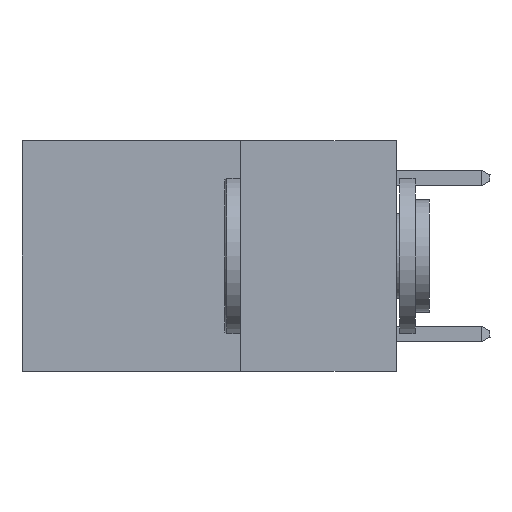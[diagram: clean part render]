
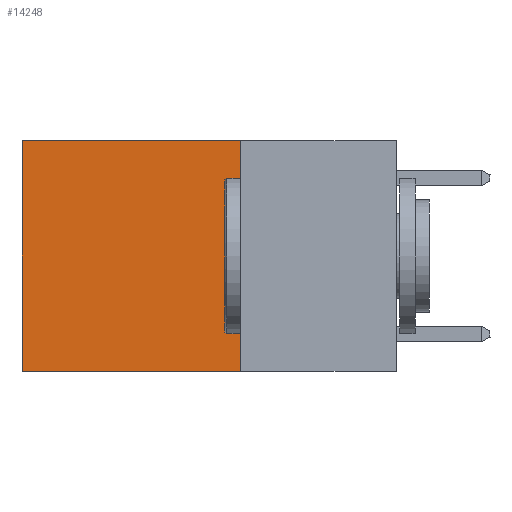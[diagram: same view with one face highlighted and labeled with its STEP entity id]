
A CAD part, left-side view. The second image highlights one B-rep face of the part: STEP entity #14248.
In plain terms, the highlighted planar face has unit normal (-1, 0, 0).
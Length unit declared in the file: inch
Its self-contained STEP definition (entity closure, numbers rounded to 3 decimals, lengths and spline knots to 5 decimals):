
#1672 = EDGE_CURVE ( 'NONE', #14517, #18573, #16495, .T. ) ;
#2757 = LINE ( 'NONE', #18654, #20896 ) ;
#2810 = LINE ( 'NONE', #10852, #20911 ) ;
#2947 = CARTESIAN_POINT ( 'NONE',  ( 0.2625, 0.25, -0.37 ) ) ;
#3266 = DIRECTION ( 'NONE',  ( 0., 0., -1. ) ) ;
#4564 = VERTEX_POINT ( 'NONE', #9710 ) ;
#4929 = DIRECTION ( 'NONE',  ( 0., 1., 0. ) ) ;
#6779 = LINE ( 'NONE', #2947, #18053 ) ;
#7297 = ORIENTED_EDGE ( 'NONE', *, *, #20606, .T. ) ;
#8660 = VERTEX_POINT ( 'NONE', #10521 ) ;
#8842 = DIRECTION ( 'NONE',  ( 0., 0., -1. ) ) ;
#9063 = DIRECTION ( 'NONE',  ( 1., 0., 0. ) ) ;
#9200 = CARTESIAN_POINT ( 'NONE',  ( 0.2625, 0.25, 0. ) ) ;
#9710 = CARTESIAN_POINT ( 'NONE',  ( 0.2625, 0.6, -0.37 ) ) ;
#10521 = CARTESIAN_POINT ( 'NONE',  ( 0.2625, 0.25, -0.37 ) ) ;
#10604 = CARTESIAN_POINT ( 'NONE',  ( 0.2625, 0.25, 0. ) ) ;
#10770 = ORIENTED_EDGE ( 'NONE', *, *, #19066, .F. ) ;
#10775 = EDGE_LOOP ( 'NONE', ( #7297, #10770, #15375, #19429 ) ) ;
#10852 = CARTESIAN_POINT ( 'NONE',  ( 0.2625, 0.6, 0. ) ) ;
#10912 = EDGE_CURVE ( 'NONE', #14517, #8660, #2757, .T. ) ;
#14248 = ADVANCED_FACE ( 'NONE', ( #19027 ), #23471, .F. ) ;
#14517 = VERTEX_POINT ( 'NONE', #10604 ) ;
#14653 = CARTESIAN_POINT ( 'NONE',  ( 0.2625, 0.25, 0. ) ) ;
#15375 = ORIENTED_EDGE ( 'NONE', *, *, #10912, .F. ) ;
#16280 = CARTESIAN_POINT ( 'NONE',  ( 0.2625, 0.6, 0. ) ) ;
#16495 = LINE ( 'NONE', #14653, #22842 ) ;
#18053 = VECTOR ( 'NONE', #20395, 39.37008 ) ;
#18573 = VERTEX_POINT ( 'NONE', #16280 ) ;
#18654 = CARTESIAN_POINT ( 'NONE',  ( 0.2625, 0.25, 0. ) ) ;
#18839 = DIRECTION ( 'NONE',  ( 0., 0., -1. ) ) ;
#19027 = FACE_OUTER_BOUND ( 'NONE', #10775, .T. ) ;
#19066 = EDGE_CURVE ( 'NONE', #8660, #4564, #6779, .T. ) ;
#19429 = ORIENTED_EDGE ( 'NONE', *, *, #1672, .T. ) ;
#20395 = DIRECTION ( 'NONE',  ( 0., 1., 0. ) ) ;
#20606 = EDGE_CURVE ( 'NONE', #18573, #4564, #2810, .T. ) ;
#20896 = VECTOR ( 'NONE', #8842, 39.37008 ) ;
#20911 = VECTOR ( 'NONE', #18839, 39.37008 ) ;
#22842 = VECTOR ( 'NONE', #4929, 39.37008 ) ;
#23471 = PLANE ( 'NONE',  #25487 ) ;
#25487 = AXIS2_PLACEMENT_3D ( 'NONE', #9200, #9063, #3266 ) ;
